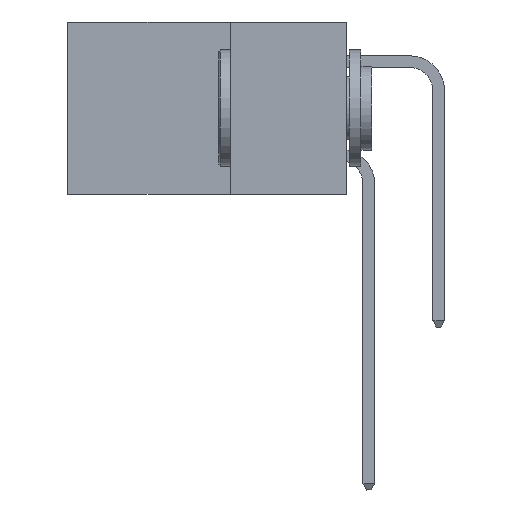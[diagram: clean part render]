
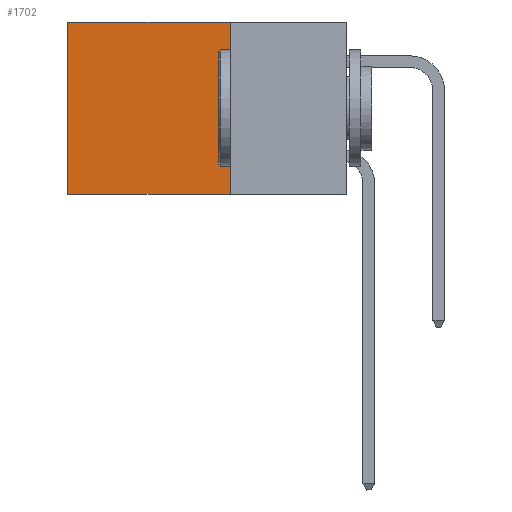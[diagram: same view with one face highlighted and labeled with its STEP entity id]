
A CAD part, left-side view. The second image highlights one B-rep face of the part: STEP entity #1702.
In plain terms, the highlighted planar face has unit normal (-1, 0, 0).
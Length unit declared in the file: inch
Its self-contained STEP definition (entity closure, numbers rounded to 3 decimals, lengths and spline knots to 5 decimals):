
#1523 = EDGE_CURVE ( 'NONE', #14228, #13912, #1628, .T. ) ;
#1628 = LINE ( 'NONE', #4563, #14012 ) ;
#1702 = ADVANCED_FACE ( 'NONE', ( #19645 ), #2273, .F. ) ;
#1773 = ORIENTED_EDGE ( 'NONE', *, *, #1523, .T. ) ;
#2134 = DIRECTION ( 'NONE',  ( 1., 0., 0. ) ) ;
#2273 = PLANE ( 'NONE',  #3576 ) ;
#3269 = VECTOR ( 'NONE', #4707, 39.37008 ) ;
#3486 = EDGE_CURVE ( 'NONE', #19936, #19590, #12419, .T. ) ;
#3576 = AXIS2_PLACEMENT_3D ( 'NONE', #10603, #2134, #3756 ) ;
#3754 = ORIENTED_EDGE ( 'NONE', *, *, #8553, .F. ) ;
#3756 = DIRECTION ( 'NONE',  ( 0., 0., -1. ) ) ;
#3976 = VECTOR ( 'NONE', #20282, 39.37008 ) ;
#4563 = CARTESIAN_POINT ( 'NONE',  ( 0.2875, 0.6, 0. ) ) ;
#4707 = DIRECTION ( 'NONE',  ( 0., 1., 0. ) ) ;
#5734 = CARTESIAN_POINT ( 'NONE',  ( 0.2875, 0.25, -0.37 ) ) ;
#5800 = CARTESIAN_POINT ( 'NONE',  ( 0.2875, 0.25, -0.37 ) ) ;
#6817 = DIRECTION ( 'NONE',  ( 0., 0., -1. ) ) ;
#8515 = ORIENTED_EDGE ( 'NONE', *, *, #21617, .T. ) ;
#8553 = EDGE_CURVE ( 'NONE', #19590, #13912, #15739, .T. ) ;
#10354 = VECTOR ( 'NONE', #13998, 39.37008 ) ;
#10603 = CARTESIAN_POINT ( 'NONE',  ( 0.2875, 0.25, 0. ) ) ;
#11719 = LINE ( 'NONE', #14702, #3269 ) ;
#12419 = LINE ( 'NONE', #20334, #3976 ) ;
#13912 = VERTEX_POINT ( 'NONE', #14351 ) ;
#13998 = DIRECTION ( 'NONE',  ( 0., 1., 0. ) ) ;
#14012 = VECTOR ( 'NONE', #6817, 39.37008 ) ;
#14228 = VERTEX_POINT ( 'NONE', #19991 ) ;
#14351 = CARTESIAN_POINT ( 'NONE',  ( 0.2875, 0.6, -0.37 ) ) ;
#14702 = CARTESIAN_POINT ( 'NONE',  ( 0.2875, 0.25, 0. ) ) ;
#15046 = CARTESIAN_POINT ( 'NONE',  ( 0.2875, 0.25, 0. ) ) ;
#15739 = LINE ( 'NONE', #5734, #10354 ) ;
#17382 = EDGE_LOOP ( 'NONE', ( #1773, #3754, #18696, #8515 ) ) ;
#18696 = ORIENTED_EDGE ( 'NONE', *, *, #3486, .F. ) ;
#19590 = VERTEX_POINT ( 'NONE', #5800 ) ;
#19645 = FACE_OUTER_BOUND ( 'NONE', #17382, .T. ) ;
#19936 = VERTEX_POINT ( 'NONE', #15046 ) ;
#19991 = CARTESIAN_POINT ( 'NONE',  ( 0.2875, 0.6, 0. ) ) ;
#20282 = DIRECTION ( 'NONE',  ( 0., 0., -1. ) ) ;
#20334 = CARTESIAN_POINT ( 'NONE',  ( 0.2875, 0.25, 0. ) ) ;
#21617 = EDGE_CURVE ( 'NONE', #19936, #14228, #11719, .T. ) ;
